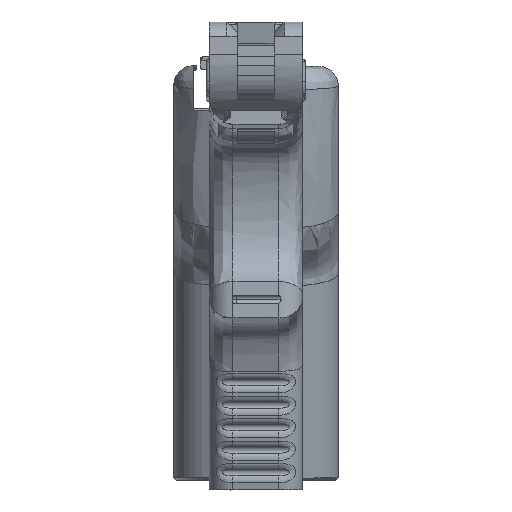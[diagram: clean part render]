
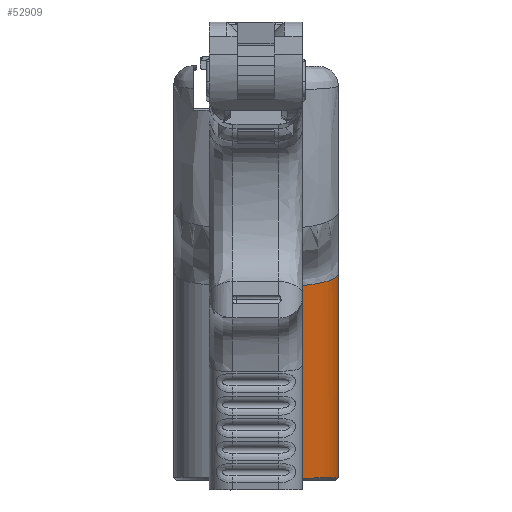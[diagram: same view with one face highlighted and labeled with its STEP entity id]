
A CAD part, front view. The second image highlights one B-rep face of the part: STEP entity #52909.
In plain terms, the highlighted cylindrical face has radius 8 mm (diameter 16 mm), a partial arc.
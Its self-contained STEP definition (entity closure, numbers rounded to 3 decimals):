
#3961=B_SPLINE_CURVE_WITH_KNOTS('',3,(#109485,#109486,#109487,#109488,#109489),
 .UNSPECIFIED.,.F.,.F.,(4,1,4),(-1.554,-0.801,-0.236),
 .UNSPECIFIED.);
#7463=FACE_OUTER_BOUND('',#10449,.T.);
#10449=EDGE_LOOP('',(#47104,#47105,#47106,#47107));
#14510=LINE('',#108929,#19326);
#14548=LINE('',#109580,#19364);
#19326=VECTOR('',#63003,8.);
#19364=VECTOR('',#63153,10.);
#21316=CIRCLE('',#55389,8.);
#25483=VERTEX_POINT('',#108888);
#25484=VERTEX_POINT('',#108928);
#25530=VERTEX_POINT('',#109475);
#25540=VERTEX_POINT('',#109578);
#32810=EDGE_CURVE('',#25484,#25483,#14510,.T.);
#32884=EDGE_CURVE('',#25484,#25530,#3961,.T.);
#32897=EDGE_CURVE('',#25483,#25540,#21316,.T.);
#32898=EDGE_CURVE('',#25530,#25540,#14548,.T.);
#47104=ORIENTED_EDGE('',*,*,#32884,.F.);
#47105=ORIENTED_EDGE('',*,*,#32810,.T.);
#47106=ORIENTED_EDGE('',*,*,#32897,.T.);
#47107=ORIENTED_EDGE('',*,*,#32898,.F.);
#50633=CYLINDRICAL_SURFACE('',#55388,8.);
#52909=ADVANCED_FACE('',(#7463),#50633,.T.);
#55388=AXIS2_PLACEMENT_3D('',#109577,#63149,#63150);
#55389=AXIS2_PLACEMENT_3D('',#109579,#63151,#63152);
#63003=DIRECTION('',(0.264,0.,0.965));
#63149=DIRECTION('center_axis',(0.264,0.,0.965));
#63150=DIRECTION('ref_axis',(0.937,0.238,-0.256));
#63151=DIRECTION('center_axis',(-0.264,0.,-0.965));
#63152=DIRECTION('ref_axis',(0.,1.,0.));
#63153=DIRECTION('',(0.264,0.,0.965));
#108888=CARTESIAN_POINT('',(22.511,6.1,-2.306));
#108928=CARTESIAN_POINT('',(13.083,6.1,-36.82));
#108929=CARTESIAN_POINT('',(13.505,6.1,-35.272));
#109475=CARTESIAN_POINT('',(21.134,0.,-36.837));
#109485=CARTESIAN_POINT('Ctrl Pts',(13.083,6.1,-36.82));
#109486=CARTESIAN_POINT('Ctrl Pts',(15.166,6.1,-36.82));
#109487=CARTESIAN_POINT('Ctrl Pts',(18.818,4.706,-36.827));
#109488=CARTESIAN_POINT('Ctrl Pts',(20.757,1.488,-36.835));
#109489=CARTESIAN_POINT('Ctrl Pts',(21.134,0.,
-36.837));
#109577=CARTESIAN_POINT('Origin',(13.505,-1.9,-35.272));
#109578=CARTESIAN_POINT('',(30.008,0.,-4.354));
#109579=CARTESIAN_POINT('Origin',(22.511,-1.9,-2.306));
#109580=CARTESIAN_POINT('',(21.002,0.,-37.32));
